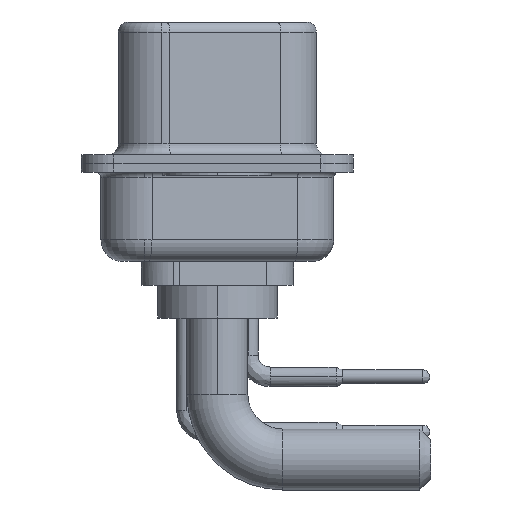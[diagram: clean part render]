
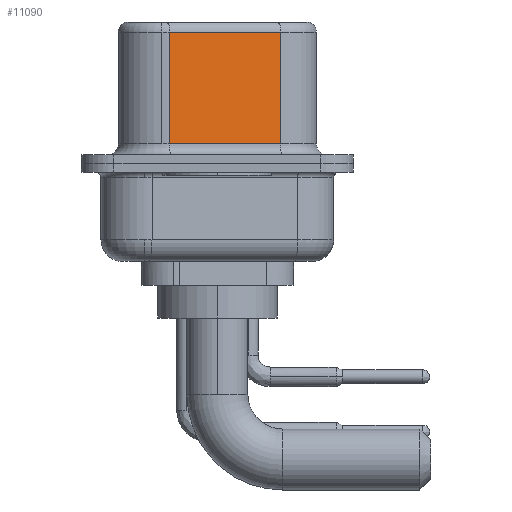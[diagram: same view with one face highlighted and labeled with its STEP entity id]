
A CAD part, left-side view. The second image highlights one B-rep face of the part: STEP entity #11090.
In plain terms, the highlighted planar face has unit normal (-0.985, -0.174, 0).
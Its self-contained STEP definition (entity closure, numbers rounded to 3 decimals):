
#142 = EDGE_CURVE ( 'NONE', #2231, #18525, #15885, .T. ) ;
#1412 = CARTESIAN_POINT ( 'NONE',  ( 4.58, -2.897, 0.9 ) ) ;
#1611 = CARTESIAN_POINT ( 'NONE',  ( 4.58, -2.897, 6.02 ) ) ;
#1633 = DIRECTION ( 'NONE',  ( -0.174, 0.985, 0. ) ) ;
#1974 = VECTOR ( 'NONE', #11368, 1000. ) ;
#2044 = DIRECTION ( 'NONE',  ( -0.174, 0.985, 0. ) ) ;
#2216 = EDGE_CURVE ( 'NONE', #8581, #20586, #20898, .T. ) ;
#2231 = VERTEX_POINT ( 'NONE', #12530 ) ;
#2758 = EDGE_CURVE ( 'NONE', #8581, #2231, #14867, .T. ) ;
#3583 = CARTESIAN_POINT ( 'NONE',  ( 4.58, -2.897, 6.52 ) ) ;
#3657 = VECTOR ( 'NONE', #1633, 1000. ) ;
#4177 = CARTESIAN_POINT ( 'NONE',  ( 3.68, 2.203, 6.52 ) ) ;
#4346 = DIRECTION ( 'NONE',  ( 0., 0., -1. ) ) ;
#5245 = FACE_OUTER_BOUND ( 'NONE', #20726, .T. ) ;
#5777 = EDGE_CURVE ( 'NONE', #18525, #20586, #19723, .T. ) ;
#6012 = CARTESIAN_POINT ( 'NONE',  ( 3.68, 2.203, 0.9 ) ) ;
#6719 = CARTESIAN_POINT ( 'NONE',  ( 4.58, -2.897, 6.02 ) ) ;
#7368 = AXIS2_PLACEMENT_3D ( 'NONE', #3583, #11887, #2044 ) ;
#8581 = VERTEX_POINT ( 'NONE', #1611 ) ;
#9295 = ORIENTED_EDGE ( 'NONE', *, *, #142, .T. ) ;
#9826 = CARTESIAN_POINT ( 'NONE',  ( 4.58, -2.897, 0.9 ) ) ;
#9940 = VECTOR ( 'NONE', #17849, 1000. ) ;
#11090 = ADVANCED_FACE ( 'NONE', ( #5245 ), #13527, .F. ) ;
#11368 = DIRECTION ( 'NONE',  ( 0.174, -0.985, 0. ) ) ;
#11887 = DIRECTION ( 'NONE',  ( 0.985, 0.174, 0. ) ) ;
#12530 = CARTESIAN_POINT ( 'NONE',  ( 3.68, 2.203, 6.02 ) ) ;
#13527 = PLANE ( 'NONE',  #7368 ) ;
#14867 = LINE ( 'NONE', #6719, #3657 ) ;
#15885 = LINE ( 'NONE', #4177, #9940 ) ;
#17590 = CARTESIAN_POINT ( 'NONE',  ( 4.58, -2.897, 6.52 ) ) ;
#17849 = DIRECTION ( 'NONE',  ( 0., 0., -1. ) ) ;
#18525 = VERTEX_POINT ( 'NONE', #6012 ) ;
#18789 = VECTOR ( 'NONE', #4346, 1000. ) ;
#19078 = ORIENTED_EDGE ( 'NONE', *, *, #2216, .F. ) ;
#19723 = LINE ( 'NONE', #9826, #1974 ) ;
#20371 = ORIENTED_EDGE ( 'NONE', *, *, #5777, .T. ) ;
#20508 = ORIENTED_EDGE ( 'NONE', *, *, #2758, .T. ) ;
#20586 = VERTEX_POINT ( 'NONE', #1412 ) ;
#20726 = EDGE_LOOP ( 'NONE', ( #19078, #20508, #9295, #20371 ) ) ;
#20898 = LINE ( 'NONE', #17590, #18789 ) ;
